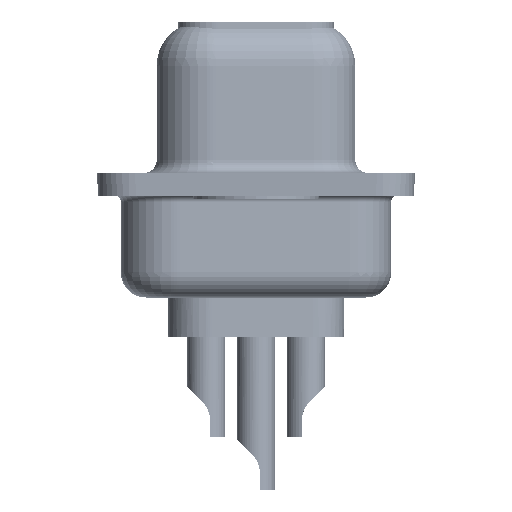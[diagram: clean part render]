
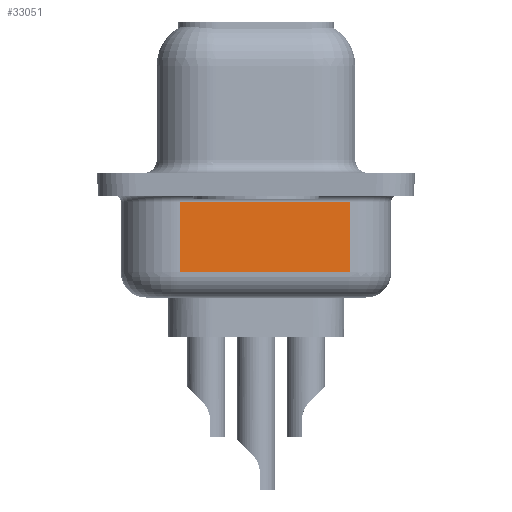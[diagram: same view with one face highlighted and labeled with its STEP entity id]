
A CAD part, left-side view. The second image highlights one B-rep face of the part: STEP entity #33051.
In plain terms, the highlighted planar face has unit normal (-0.985, -0.174, 0).
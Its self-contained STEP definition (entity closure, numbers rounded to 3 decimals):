
#1628 = EDGE_CURVE ( 'NONE', #19221, #10300, #30173, .T. ) ;
#2603 = ORIENTED_EDGE ( 'NONE', *, *, #25801, .T. ) ;
#3754 = FACE_OUTER_BOUND ( 'NONE', #16019, .T. ) ;
#4029 = CARTESIAN_POINT ( 'NONE',  ( 3.13, 3.028, -0.7 ) ) ;
#4980 = LINE ( 'NONE', #10684, #41049 ) ;
#5318 = CARTESIAN_POINT ( 'NONE',  ( 3.13, 3.028, -3.5 ) ) ;
#7135 = VECTOR ( 'NONE', #33744, 1000. ) ;
#7137 = CARTESIAN_POINT ( 'NONE',  ( 3.13, 3.028, -4.5 ) ) ;
#7249 = LINE ( 'NONE', #26757, #7883 ) ;
#7601 = AXIS2_PLACEMENT_3D ( 'NONE', #7137, #10092, #13209 ) ;
#7883 = VECTOR ( 'NONE', #36375, 1000. ) ;
#10092 = DIRECTION ( 'NONE',  ( 0.985, 0.174, 0. ) ) ;
#10300 = VERTEX_POINT ( 'NONE', #38076 ) ;
#10684 = CARTESIAN_POINT ( 'NONE',  ( 3.13, 3.028, -3.5 ) ) ;
#13209 = DIRECTION ( 'NONE',  ( -0.174, 0.985, 0. ) ) ;
#13781 = CARTESIAN_POINT ( 'NONE',  ( 3.13, 3.028, -0.7 ) ) ;
#15243 = ORIENTED_EDGE ( 'NONE', *, *, #1628, .T. ) ;
#16019 = EDGE_LOOP ( 'NONE', ( #26629, #2603, #15243, #22489 ) ) ;
#19221 = VERTEX_POINT ( 'NONE', #21205 ) ;
#19578 = VECTOR ( 'NONE', #26290, 1000. ) ;
#20948 = CARTESIAN_POINT ( 'NONE',  ( 4.321, -3.722, -4.5 ) ) ;
#21163 = VERTEX_POINT ( 'NONE', #13781 ) ;
#21205 = CARTESIAN_POINT ( 'NONE',  ( 4.321, -3.722, -3.5 ) ) ;
#22489 = ORIENTED_EDGE ( 'NONE', *, *, #32543, .T. ) ;
#25801 = EDGE_CURVE ( 'NONE', #32302, #19221, #4980, .T. ) ;
#26290 = DIRECTION ( 'NONE',  ( -0.174, 0.985, 0. ) ) ;
#26629 = ORIENTED_EDGE ( 'NONE', *, *, #37034, .F. ) ;
#26757 = CARTESIAN_POINT ( 'NONE',  ( 3.13, 3.028, -4.5 ) ) ;
#30173 = LINE ( 'NONE', #20948, #7135 ) ;
#30560 = DIRECTION ( 'NONE',  ( 0.174, -0.985, 0. ) ) ;
#32302 = VERTEX_POINT ( 'NONE', #5318 ) ;
#32543 = EDGE_CURVE ( 'NONE', #10300, #21163, #38845, .T. ) ;
#33051 = ADVANCED_FACE ( 'NONE', ( #3754 ), #35648, .F. ) ;
#33744 = DIRECTION ( 'NONE',  ( 0., 0., 1. ) ) ;
#35648 = PLANE ( 'NONE',  #7601 ) ;
#36375 = DIRECTION ( 'NONE',  ( 0., 0., 1. ) ) ;
#37034 = EDGE_CURVE ( 'NONE', #32302, #21163, #7249, .T. ) ;
#38076 = CARTESIAN_POINT ( 'NONE',  ( 4.321, -3.722, -0.7 ) ) ;
#38845 = LINE ( 'NONE', #4029, #19578 ) ;
#41049 = VECTOR ( 'NONE', #30560, 1000. ) ;
